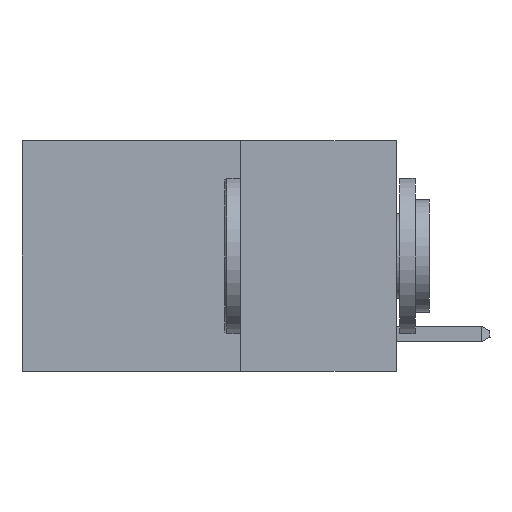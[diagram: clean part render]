
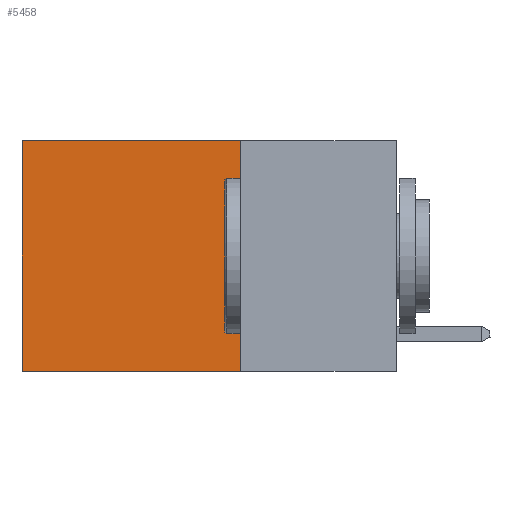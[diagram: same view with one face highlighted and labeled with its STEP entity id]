
A CAD part, left-side view. The second image highlights one B-rep face of the part: STEP entity #5458.
In plain terms, the highlighted planar face has unit normal (-1, 0, 0).
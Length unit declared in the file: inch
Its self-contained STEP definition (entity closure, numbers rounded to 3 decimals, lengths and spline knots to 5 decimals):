
#88 = CARTESIAN_POINT ( 'NONE',  ( 0.2625, 0.25, -0.37 ) ) ;
#813 = FACE_OUTER_BOUND ( 'NONE', #8009, .T. ) ;
#1285 = ORIENTED_EDGE ( 'NONE', *, *, #3598, .T. ) ;
#2989 = LINE ( 'NONE', #3190, #5953 ) ;
#3103 = DIRECTION ( 'NONE',  ( 0., 0., -1. ) ) ;
#3190 = CARTESIAN_POINT ( 'NONE',  ( 0.2625, 0.6, 0. ) ) ;
#3598 = EDGE_CURVE ( 'NONE', #6209, #7851, #2989, .T. ) ;
#4507 = CARTESIAN_POINT ( 'NONE',  ( 0.2625, 0.6, 0. ) ) ;
#4634 = DIRECTION ( 'NONE',  ( 0., 1., 0. ) ) ;
#5458 = ADVANCED_FACE ( 'NONE', ( #813 ), #10494, .F. ) ;
#5570 = VECTOR ( 'NONE', #14023, 39.37008 ) ;
#5616 = EDGE_CURVE ( 'NONE', #8073, #7851, #8197, .T. ) ;
#5953 = VECTOR ( 'NONE', #9369, 39.37008 ) ;
#6000 = VERTEX_POINT ( 'NONE', #6624 ) ;
#6209 = VERTEX_POINT ( 'NONE', #4507 ) ;
#6624 = CARTESIAN_POINT ( 'NONE',  ( 0.2625, 0.25, 0. ) ) ;
#7851 = VERTEX_POINT ( 'NONE', #13900 ) ;
#8009 = EDGE_LOOP ( 'NONE', ( #1285, #8795, #15141, #10511 ) ) ;
#8073 = VERTEX_POINT ( 'NONE', #88 ) ;
#8197 = LINE ( 'NONE', #13170, #14209 ) ;
#8795 = ORIENTED_EDGE ( 'NONE', *, *, #5616, .F. ) ;
#9199 = CARTESIAN_POINT ( 'NONE',  ( 0.2625, 0.25, 0. ) ) ;
#9293 = CARTESIAN_POINT ( 'NONE',  ( 0.2625, 0.25, 0. ) ) ;
#9369 = DIRECTION ( 'NONE',  ( 0., 0., -1. ) ) ;
#10494 = PLANE ( 'NONE',  #15713 ) ;
#10511 = ORIENTED_EDGE ( 'NONE', *, *, #14484, .T. ) ;
#10678 = DIRECTION ( 'NONE',  ( 0., 0., -1. ) ) ;
#11806 = VECTOR ( 'NONE', #10678, 39.37008 ) ;
#11834 = CARTESIAN_POINT ( 'NONE',  ( 0.2625, 0.25, 0. ) ) ;
#12033 = LINE ( 'NONE', #9199, #5570 ) ;
#12863 = DIRECTION ( 'NONE',  ( 1., 0., 0. ) ) ;
#13170 = CARTESIAN_POINT ( 'NONE',  ( 0.2625, 0.25, -0.37 ) ) ;
#13900 = CARTESIAN_POINT ( 'NONE',  ( 0.2625, 0.6, -0.37 ) ) ;
#14023 = DIRECTION ( 'NONE',  ( 0., 1., 0. ) ) ;
#14209 = VECTOR ( 'NONE', #4634, 39.37008 ) ;
#14484 = EDGE_CURVE ( 'NONE', #6000, #6209, #12033, .T. ) ;
#14938 = LINE ( 'NONE', #11834, #11806 ) ;
#15141 = ORIENTED_EDGE ( 'NONE', *, *, #16012, .F. ) ;
#15713 = AXIS2_PLACEMENT_3D ( 'NONE', #9293, #12863, #3103 ) ;
#16012 = EDGE_CURVE ( 'NONE', #6000, #8073, #14938, .T. ) ;
